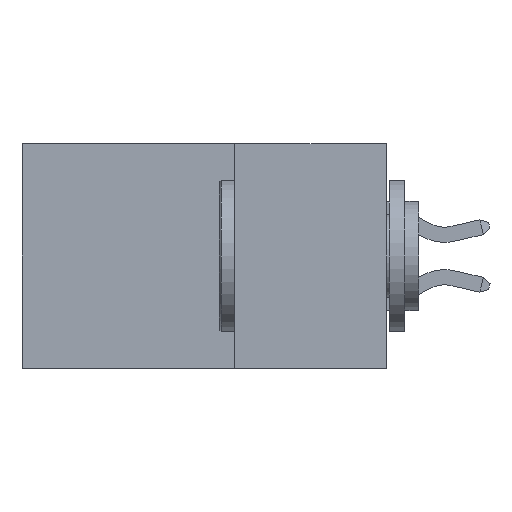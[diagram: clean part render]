
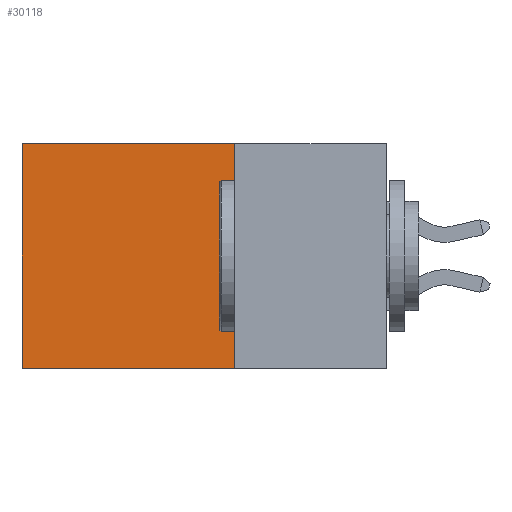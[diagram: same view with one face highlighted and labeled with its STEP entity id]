
A CAD part, left-side view. The second image highlights one B-rep face of the part: STEP entity #30118.
In plain terms, the highlighted planar face has unit normal (-1, 0, 0).
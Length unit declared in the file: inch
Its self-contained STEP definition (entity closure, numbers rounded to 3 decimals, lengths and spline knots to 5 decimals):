
#693 = CARTESIAN_POINT ( 'NONE',  ( 0.298, 0.25, 0. ) ) ;
#1729 = VECTOR ( 'NONE', #11139, 39.37008 ) ;
#2580 = CARTESIAN_POINT ( 'NONE',  ( 0.298, 0.25, 0. ) ) ;
#5212 = PLANE ( 'NONE',  #21761 ) ;
#5511 = CARTESIAN_POINT ( 'NONE',  ( 0.298, 0.6, 0. ) ) ;
#6000 = ORIENTED_EDGE ( 'NONE', *, *, #13044, .F. ) ;
#6374 = EDGE_LOOP ( 'NONE', ( #9953, #6000, #14337, #24966 ) ) ;
#6469 = CARTESIAN_POINT ( 'NONE',  ( 0.298, 0.6, 0. ) ) ;
#8194 = LINE ( 'NONE', #6469, #23074 ) ;
#8432 = DIRECTION ( 'NONE',  ( 0., 0., -1. ) ) ;
#8711 = CARTESIAN_POINT ( 'NONE',  ( 0.298, 0.25, 0. ) ) ;
#8910 = EDGE_CURVE ( 'NONE', #13014, #12771, #8194, .T. ) ;
#9953 = ORIENTED_EDGE ( 'NONE', *, *, #8910, .T. ) ;
#10177 = VERTEX_POINT ( 'NONE', #16368 ) ;
#11139 = DIRECTION ( 'NONE',  ( 0., 1., 0. ) ) ;
#11751 = EDGE_CURVE ( 'NONE', #28393, #13014, #23680, .T. ) ;
#12771 = VERTEX_POINT ( 'NONE', #31249 ) ;
#13014 = VERTEX_POINT ( 'NONE', #5511 ) ;
#13044 = EDGE_CURVE ( 'NONE', #10177, #12771, #16964, .T. ) ;
#13366 = DIRECTION ( 'NONE',  ( 1., 0., 0. ) ) ;
#14021 = EDGE_CURVE ( 'NONE', #28393, #10177, #32052, .T. ) ;
#14139 = DIRECTION ( 'NONE',  ( 0., 1., 0. ) ) ;
#14337 = ORIENTED_EDGE ( 'NONE', *, *, #14021, .F. ) ;
#16368 = CARTESIAN_POINT ( 'NONE',  ( 0.298, 0.25, -0.37 ) ) ;
#16964 = LINE ( 'NONE', #19352, #1729 ) ;
#18458 = CARTESIAN_POINT ( 'NONE',  ( 0.298, 0.25, 0. ) ) ;
#19352 = CARTESIAN_POINT ( 'NONE',  ( 0.298, 0.25, -0.37 ) ) ;
#19978 = FACE_OUTER_BOUND ( 'NONE', #6374, .T. ) ;
#21761 = AXIS2_PLACEMENT_3D ( 'NONE', #18458, #13366, #23778 ) ;
#23074 = VECTOR ( 'NONE', #8432, 39.37008 ) ;
#23680 = LINE ( 'NONE', #8711, #25338 ) ;
#23778 = DIRECTION ( 'NONE',  ( 0., 0., -1. ) ) ;
#24966 = ORIENTED_EDGE ( 'NONE', *, *, #11751, .T. ) ;
#25338 = VECTOR ( 'NONE', #14139, 39.37008 ) ;
#26326 = VECTOR ( 'NONE', #32957, 39.37008 ) ;
#28393 = VERTEX_POINT ( 'NONE', #2580 ) ;
#30118 = ADVANCED_FACE ( 'NONE', ( #19978 ), #5212, .F. ) ;
#31249 = CARTESIAN_POINT ( 'NONE',  ( 0.298, 0.6, -0.37 ) ) ;
#32052 = LINE ( 'NONE', #693, #26326 ) ;
#32957 = DIRECTION ( 'NONE',  ( 0., 0., -1. ) ) ;
